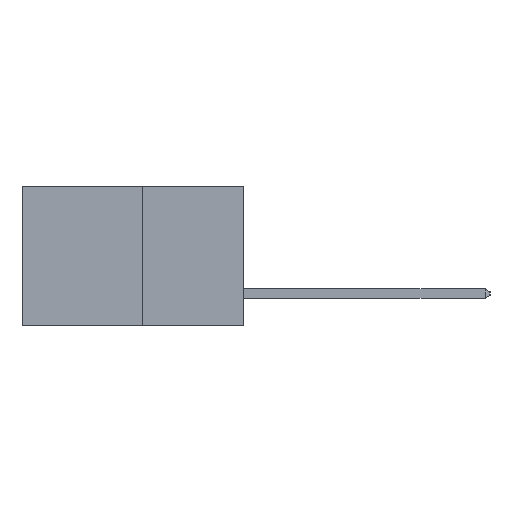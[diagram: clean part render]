
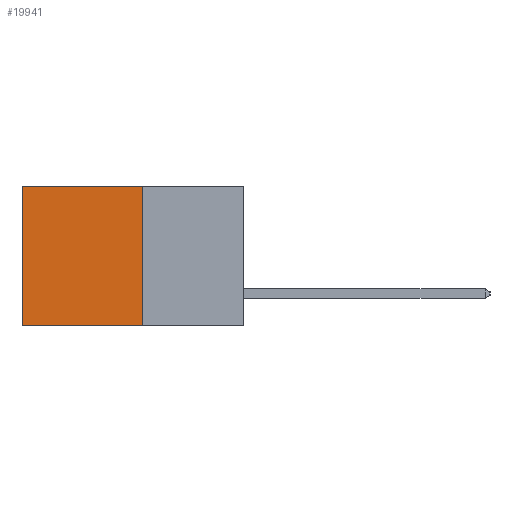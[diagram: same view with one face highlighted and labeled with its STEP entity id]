
A CAD part, left-side view. The second image highlights one B-rep face of the part: STEP entity #19941.
In plain terms, the highlighted planar face has unit normal (-1, 0, 0).
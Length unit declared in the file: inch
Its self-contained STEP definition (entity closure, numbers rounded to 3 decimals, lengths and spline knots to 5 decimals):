
#643 = LINE ( 'NONE', #7319, #18329 ) ;
#921 = DIRECTION ( 'NONE',  ( 0., 0., -1. ) ) ;
#1393 = LINE ( 'NONE', #15492, #17616 ) ;
#1591 = EDGE_CURVE ( 'NONE', #10052, #12575, #3984, .T. ) ;
#3198 = CARTESIAN_POINT ( 'NONE',  ( 0.277, 0.59, 0. ) ) ;
#3707 = ORIENTED_EDGE ( 'NONE', *, *, #11074, .F. ) ;
#3786 = VERTEX_POINT ( 'NONE', #5667 ) ;
#3984 = LINE ( 'NONE', #10394, #11931 ) ;
#4849 = CARTESIAN_POINT ( 'NONE',  ( 0.277, 0.27, -0.37 ) ) ;
#5446 = CARTESIAN_POINT ( 'NONE',  ( 0.277, 0.27, -0.37 ) ) ;
#5667 = CARTESIAN_POINT ( 'NONE',  ( 0.277, 0.27, -0.37 ) ) ;
#5798 = CARTESIAN_POINT ( 'NONE',  ( 0.277, 0.27, 0. ) ) ;
#6483 = EDGE_LOOP ( 'NONE', ( #8707, #3707, #19158, #10208 ) ) ;
#7319 = CARTESIAN_POINT ( 'NONE',  ( 0.277, 0.27, -0.37 ) ) ;
#7460 = VECTOR ( 'NONE', #13452, 39.37008 ) ;
#8076 = DIRECTION ( 'NONE',  ( 0., 0., -1. ) ) ;
#8370 = FACE_OUTER_BOUND ( 'NONE', #6483, .T. ) ;
#8707 = ORIENTED_EDGE ( 'NONE', *, *, #1591, .T. ) ;
#10052 = VERTEX_POINT ( 'NONE', #3198 ) ;
#10208 = ORIENTED_EDGE ( 'NONE', *, *, #14096, .T. ) ;
#10394 = CARTESIAN_POINT ( 'NONE',  ( 0.277, 0.59, -0.37 ) ) ;
#11020 = DIRECTION ( 'NONE',  ( 0., 0., -1. ) ) ;
#11074 = EDGE_CURVE ( 'NONE', #3786, #12575, #16803, .T. ) ;
#11931 = VECTOR ( 'NONE', #11020, 39.37008 ) ;
#12575 = VERTEX_POINT ( 'NONE', #19333 ) ;
#12905 = AXIS2_PLACEMENT_3D ( 'NONE', #4849, #17435, #8076 ) ;
#13452 = DIRECTION ( 'NONE',  ( 0., 1., 0. ) ) ;
#13941 = EDGE_CURVE ( 'NONE', #14631, #3786, #643, .T. ) ;
#14096 = EDGE_CURVE ( 'NONE', #14631, #10052, #1393, .T. ) ;
#14402 = PLANE ( 'NONE',  #12905 ) ;
#14631 = VERTEX_POINT ( 'NONE', #5798 ) ;
#15492 = CARTESIAN_POINT ( 'NONE',  ( 0.277, 0.27, 0. ) ) ;
#15552 = DIRECTION ( 'NONE',  ( 0., 1., 0. ) ) ;
#16803 = LINE ( 'NONE', #5446, #7460 ) ;
#17435 = DIRECTION ( 'NONE',  ( 1., 0., 0. ) ) ;
#17616 = VECTOR ( 'NONE', #15552, 39.37008 ) ;
#18329 = VECTOR ( 'NONE', #921, 39.37008 ) ;
#19158 = ORIENTED_EDGE ( 'NONE', *, *, #13941, .F. ) ;
#19333 = CARTESIAN_POINT ( 'NONE',  ( 0.277, 0.59, -0.37 ) ) ;
#19941 = ADVANCED_FACE ( 'NONE', ( #8370 ), #14402, .F. ) ;
